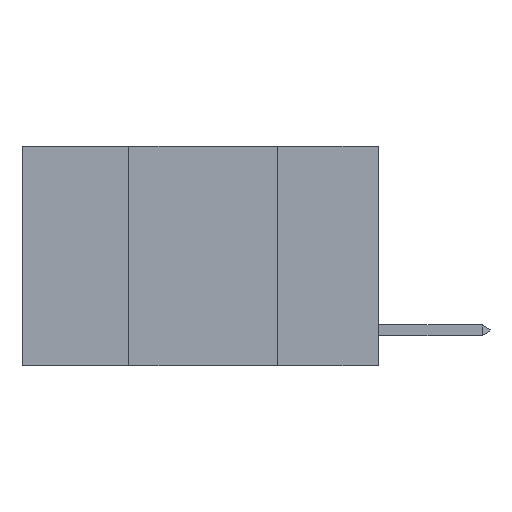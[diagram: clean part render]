
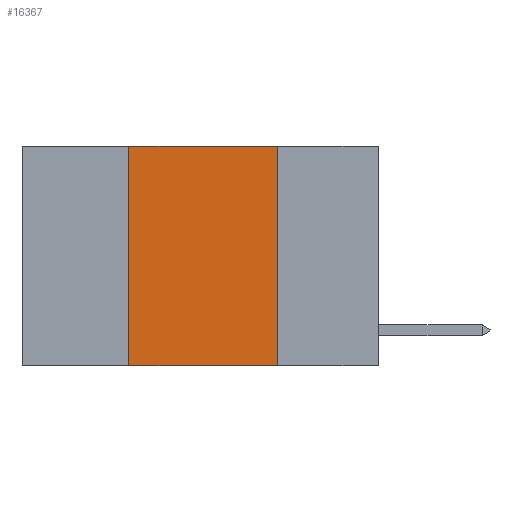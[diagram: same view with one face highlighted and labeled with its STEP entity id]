
A CAD part, left-side view. The second image highlights one B-rep face of the part: STEP entity #16367.
In plain terms, the highlighted planar face has unit normal (-1, 0, 0).
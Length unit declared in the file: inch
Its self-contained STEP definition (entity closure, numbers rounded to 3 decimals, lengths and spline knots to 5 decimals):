
#41 = FACE_OUTER_BOUND ( 'NONE', #14293, .T. ) ;
#1027 = VECTOR ( 'NONE', #15407, 39.37008 ) ;
#1942 = LINE ( 'NONE', #16931, #10731 ) ;
#2322 = VERTEX_POINT ( 'NONE', #13948 ) ;
#2499 = DIRECTION ( 'NONE',  ( 1., 0., 0. ) ) ;
#2770 = DIRECTION ( 'NONE',  ( 0., 0., -1. ) ) ;
#3993 = ORIENTED_EDGE ( 'NONE', *, *, #9078, .F. ) ;
#4847 = VERTEX_POINT ( 'NONE', #11695 ) ;
#4940 = DIRECTION ( 'NONE',  ( 0., -1., 0. ) ) ;
#4973 = EDGE_CURVE ( 'NONE', #10104, #2322, #11952, .T. ) ;
#5123 = VECTOR ( 'NONE', #5288, 39.37008 ) ;
#5288 = DIRECTION ( 'NONE',  ( 0., 0., 1. ) ) ;
#5433 = PLANE ( 'NONE',  #16663 ) ;
#5652 = VECTOR ( 'NONE', #10786, 39.37008 ) ;
#5754 = CARTESIAN_POINT ( 'NONE',  ( 0., 0.42, 0. ) ) ;
#6350 = CARTESIAN_POINT ( 'NONE',  ( 0., 0.17, -0.37 ) ) ;
#6853 = CARTESIAN_POINT ( 'NONE',  ( 0., 0.6, 0. ) ) ;
#7946 = LINE ( 'NONE', #9472, #5123 ) ;
#8896 = EDGE_CURVE ( 'NONE', #4847, #9496, #1942, .T. ) ;
#9078 = EDGE_CURVE ( 'NONE', #4847, #10104, #7946, .T. ) ;
#9383 = EDGE_CURVE ( 'NONE', #2322, #9496, #12816, .T. ) ;
#9472 = CARTESIAN_POINT ( 'NONE',  ( 0., 0.42, 0. ) ) ;
#9496 = VERTEX_POINT ( 'NONE', #6350 ) ;
#10070 = CARTESIAN_POINT ( 'NONE',  ( 0., 0.17, 0. ) ) ;
#10104 = VERTEX_POINT ( 'NONE', #5754 ) ;
#10657 = ORIENTED_EDGE ( 'NONE', *, *, #4973, .F. ) ;
#10731 = VECTOR ( 'NONE', #4940, 39.37008 ) ;
#10786 = DIRECTION ( 'NONE',  ( 0., -1., 0. ) ) ;
#11374 = ORIENTED_EDGE ( 'NONE', *, *, #8896, .T. ) ;
#11695 = CARTESIAN_POINT ( 'NONE',  ( 0., 0.42, -0.37 ) ) ;
#11952 = LINE ( 'NONE', #13215, #5652 ) ;
#12816 = LINE ( 'NONE', #10070, #1027 ) ;
#13215 = CARTESIAN_POINT ( 'NONE',  ( 0., 0.6, 0. ) ) ;
#13493 = ORIENTED_EDGE ( 'NONE', *, *, #9383, .F. ) ;
#13948 = CARTESIAN_POINT ( 'NONE',  ( 0., 0.17, 0. ) ) ;
#14293 = EDGE_LOOP ( 'NONE', ( #13493, #10657, #3993, #11374 ) ) ;
#15407 = DIRECTION ( 'NONE',  ( 0., 0., -1. ) ) ;
#16367 = ADVANCED_FACE ( 'NONE', ( #41 ), #5433, .F. ) ;
#16663 = AXIS2_PLACEMENT_3D ( 'NONE', #6853, #2499, #2770 ) ;
#16931 = CARTESIAN_POINT ( 'NONE',  ( 0., 0.6, -0.37 ) ) ;
